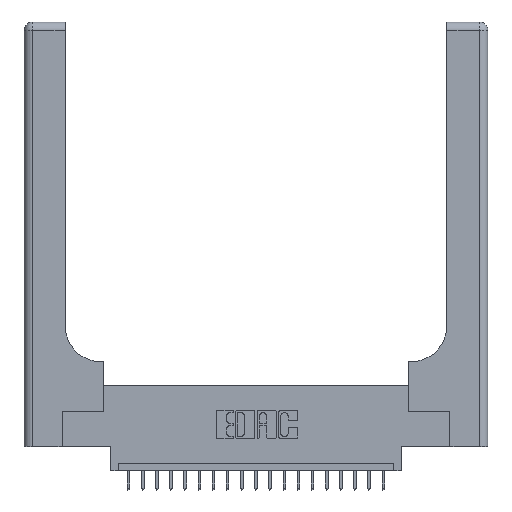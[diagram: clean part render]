
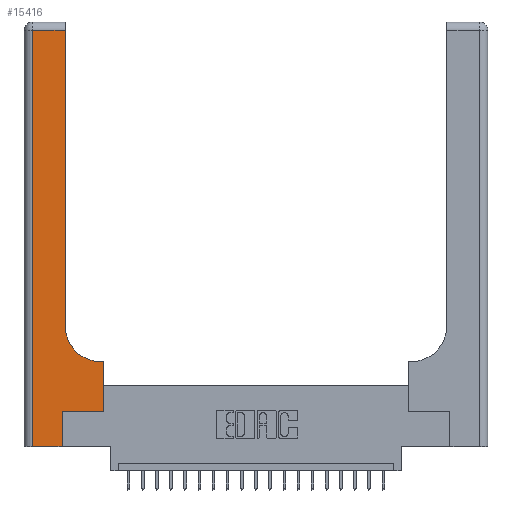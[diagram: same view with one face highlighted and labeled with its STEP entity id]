
A CAD part, top view. The second image highlights one B-rep face of the part: STEP entity #15416.
In plain terms, the highlighted planar face has unit normal (0, 0, 1).
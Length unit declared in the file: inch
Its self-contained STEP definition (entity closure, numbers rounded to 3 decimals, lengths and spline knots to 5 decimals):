
#420 = EDGE_CURVE ( 'NONE', #4806, #21667, #10014, .T. ) ;
#990 = LINE ( 'NONE', #16953, #20774 ) ;
#1192 = DIRECTION ( 'NONE',  ( 1., 0., 0. ) ) ;
#1269 = CARTESIAN_POINT ( 'NONE',  ( 0., 2.94, 0.37 ) ) ;
#1526 = EDGE_CURVE ( 'NONE', #18073, #8021, #10538, .T. ) ;
#2270 = EDGE_CURVE ( 'NONE', #6893, #18073, #12848, .T. ) ;
#2348 = CARTESIAN_POINT ( 'NONE',  ( 0.2915, 0.6, 0.37 ) ) ;
#2492 = CARTESIAN_POINT ( 'NONE',  ( 0.5415, 0.85, 0.37 ) ) ;
#3343 = VERTEX_POINT ( 'NONE', #15106 ) ;
#3503 = CARTESIAN_POINT ( 'NONE',  ( 0.2915, 0.85, 0.37 ) ) ;
#3510 = VECTOR ( 'NONE', #1192, 39.37008 ) ;
#3610 = EDGE_CURVE ( 'NONE', #8021, #3343, #20542, .T. ) ;
#4106 = LINE ( 'NONE', #2348, #8338 ) ;
#4485 = ORIENTED_EDGE ( 'NONE', *, *, #3610, .T. ) ;
#4537 = PLANE ( 'NONE',  #12031 ) ;
#4662 = CARTESIAN_POINT ( 'NONE',  ( 0.269, 0.25, 0.37 ) ) ;
#4806 = VERTEX_POINT ( 'NONE', #20646 ) ;
#4841 = CARTESIAN_POINT ( 'NONE',  ( 0.5585, 0.25, 0.37 ) ) ;
#4969 = DIRECTION ( 'NONE',  ( 0., 1., 0. ) ) ;
#6226 = EDGE_CURVE ( 'NONE', #14098, #19543, #8152, .T. ) ;
#6893 = VERTEX_POINT ( 'NONE', #14250 ) ;
#6905 = DIRECTION ( 'NONE',  ( 0., 1., 0. ) ) ;
#7022 = LINE ( 'NONE', #15938, #9841 ) ;
#8021 = VERTEX_POINT ( 'NONE', #22591 ) ;
#8152 = LINE ( 'NONE', #4662, #22278 ) ;
#8338 = VECTOR ( 'NONE', #20585, 39.37008 ) ;
#8389 = CARTESIAN_POINT ( 'NONE',  ( 0., 0., 0.37 ) ) ;
#9543 = DIRECTION ( 'NONE',  ( 0., 0., -1. ) ) ;
#9591 = DIRECTION ( 'NONE',  ( 1., 0., 0. ) ) ;
#9686 = DIRECTION ( 'NONE',  ( 0., -1., 0. ) ) ;
#9743 = EDGE_CURVE ( 'NONE', #19543, #21679, #20638, .T. ) ;
#9841 = VECTOR ( 'NONE', #6905, 39.37008 ) ;
#10014 = LINE ( 'NONE', #8389, #3510 ) ;
#10538 = LINE ( 'NONE', #17544, #18632 ) ;
#10659 = ORIENTED_EDGE ( 'NONE', *, *, #9743, .T. ) ;
#11646 = CARTESIAN_POINT ( 'NONE',  ( 0., 3., 0.37 ) ) ;
#12031 = AXIS2_PLACEMENT_3D ( 'NONE', #11646, #9543, #14869 ) ;
#12848 = CIRCLE ( 'NONE', #15783, 0.25 ) ;
#13038 = ORIENTED_EDGE ( 'NONE', *, *, #1526, .T. ) ;
#13217 = CARTESIAN_POINT ( 'NONE',  ( 0.269, 0., 0.37 ) ) ;
#13390 = FACE_OUTER_BOUND ( 'NONE', #16989, .T. ) ;
#13421 = CARTESIAN_POINT ( 'NONE',  ( 0.269, 0.25, 0.37 ) ) ;
#13958 = ORIENTED_EDGE ( 'NONE', *, *, #16339, .T. ) ;
#14098 = VERTEX_POINT ( 'NONE', #13421 ) ;
#14113 = EDGE_CURVE ( 'NONE', #3343, #4806, #990, .T. ) ;
#14144 = DIRECTION ( 'NONE',  ( 0., 1., 0. ) ) ;
#14250 = CARTESIAN_POINT ( 'NONE',  ( 0.5415, 0.6, 0.37 ) ) ;
#14839 = ORIENTED_EDGE ( 'NONE', *, *, #6226, .T. ) ;
#14869 = DIRECTION ( 'NONE',  ( -1., 0., 0. ) ) ;
#14998 = ORIENTED_EDGE ( 'NONE', *, *, #2270, .T. ) ;
#15038 = CARTESIAN_POINT ( 'NONE',  ( 0.5585, 0.6, 0.37 ) ) ;
#15106 = CARTESIAN_POINT ( 'NONE',  ( 0.06, 2.94, 0.37 ) ) ;
#15262 = DIRECTION ( 'NONE',  ( 0., 0., -1. ) ) ;
#15416 = ADVANCED_FACE ( 'NONE', ( #13390 ), #4537, .F. ) ;
#15483 = ORIENTED_EDGE ( 'NONE', *, *, #14113, .T. ) ;
#15522 = CARTESIAN_POINT ( 'NONE',  ( 0.5585, 0.25, 0.37 ) ) ;
#15620 = VECTOR ( 'NONE', #16786, 39.37008 ) ;
#15783 = AXIS2_PLACEMENT_3D ( 'NONE', #2492, #15262, #9591 ) ;
#15802 = ORIENTED_EDGE ( 'NONE', *, *, #16119, .T. ) ;
#15938 = CARTESIAN_POINT ( 'NONE',  ( 0.269, 0., 0.37 ) ) ;
#16119 = EDGE_CURVE ( 'NONE', #21667, #14098, #7022, .T. ) ;
#16339 = EDGE_CURVE ( 'NONE', #21679, #6893, #4106, .T. ) ;
#16786 = DIRECTION ( 'NONE',  ( -1., 0., 0. ) ) ;
#16953 = CARTESIAN_POINT ( 'NONE',  ( 0.06, 3., 0.37 ) ) ;
#16989 = EDGE_LOOP ( 'NONE', ( #13038, #4485, #15483, #20317, #15802, #14839, #10659, #13958, #14998 ) ) ;
#17544 = CARTESIAN_POINT ( 'NONE',  ( 0.2915, 3., 0.37 ) ) ;
#18073 = VERTEX_POINT ( 'NONE', #3503 ) ;
#18632 = VECTOR ( 'NONE', #14144, 39.37008 ) ;
#19543 = VERTEX_POINT ( 'NONE', #4841 ) ;
#20317 = ORIENTED_EDGE ( 'NONE', *, *, #420, .T. ) ;
#20542 = LINE ( 'NONE', #1269, #15620 ) ;
#20585 = DIRECTION ( 'NONE',  ( -1., 0., 0. ) ) ;
#20638 = LINE ( 'NONE', #15522, #20883 ) ;
#20646 = CARTESIAN_POINT ( 'NONE',  ( 0.06, 0., 0.37 ) ) ;
#20774 = VECTOR ( 'NONE', #9686, 39.37008 ) ;
#20883 = VECTOR ( 'NONE', #4969, 39.37008 ) ;
#21667 = VERTEX_POINT ( 'NONE', #13217 ) ;
#21679 = VERTEX_POINT ( 'NONE', #15038 ) ;
#22278 = VECTOR ( 'NONE', #22310, 39.37008 ) ;
#22310 = DIRECTION ( 'NONE',  ( 1., 0., 0. ) ) ;
#22591 = CARTESIAN_POINT ( 'NONE',  ( 0.2915, 2.94, 0.37 ) ) ;
